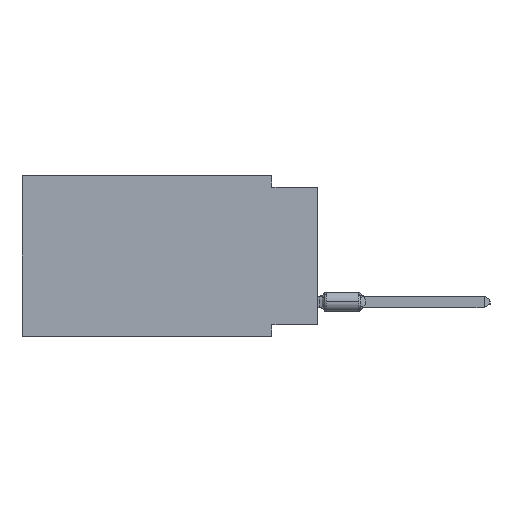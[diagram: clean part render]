
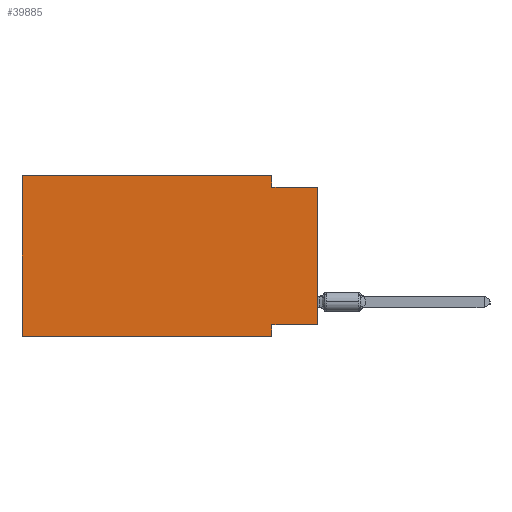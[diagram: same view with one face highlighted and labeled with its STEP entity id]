
A CAD part, left-side view. The second image highlights one B-rep face of the part: STEP entity #39885.
In plain terms, the highlighted planar face has unit normal (-1, 0, 0).
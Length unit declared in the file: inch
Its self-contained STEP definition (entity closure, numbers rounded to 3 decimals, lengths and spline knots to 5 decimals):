
#1700 = LINE ( 'NONE', #15161, #22522 ) ;
#3339 = CARTESIAN_POINT ( 'NONE',  ( 0., 0., -0.025 ) ) ;
#3641 = EDGE_CURVE ( 'NONE', #24175, #11158, #1700, .T. ) ;
#3850 = VERTEX_POINT ( 'NONE', #20729 ) ;
#4468 = EDGE_CURVE ( 'NONE', #24175, #17269, #24780, .T. ) ;
#5743 = EDGE_CURVE ( 'NONE', #25001, #36139, #16099, .T. ) ;
#5781 = DIRECTION ( 'NONE',  ( 1., 0., 0. ) ) ;
#6642 = VECTOR ( 'NONE', #9302, 39.37008 ) ;
#7160 = EDGE_CURVE ( 'NONE', #17269, #23336, #40997, .T. ) ;
#8405 = DIRECTION ( 'NONE',  ( 0., 0., -1. ) ) ;
#8498 = DIRECTION ( 'NONE',  ( 0., -1., 0. ) ) ;
#8763 = ORIENTED_EDGE ( 'NONE', *, *, #3641, .T. ) ;
#9302 = DIRECTION ( 'NONE',  ( 0., 0., -1. ) ) ;
#9422 = EDGE_CURVE ( 'NONE', #36139, #11158, #42247, .T. ) ;
#10622 = ORIENTED_EDGE ( 'NONE', *, *, #7160, .F. ) ;
#10647 = VECTOR ( 'NONE', #14175, 39.37008 ) ;
#10816 = CARTESIAN_POINT ( 'NONE',  ( 0., 0.645, 0. ) ) ;
#10922 = CARTESIAN_POINT ( 'NONE',  ( 0., 0., -0.325 ) ) ;
#10933 = CARTESIAN_POINT ( 'NONE',  ( 0., 0., 0. ) ) ;
#11158 = VERTEX_POINT ( 'NONE', #25811 ) ;
#12844 = LINE ( 'NONE', #18719, #37618 ) ;
#13560 = VECTOR ( 'NONE', #14609, 39.37008 ) ;
#13979 = EDGE_CURVE ( 'NONE', #3850, #23874, #12844, .T. ) ;
#14175 = DIRECTION ( 'NONE',  ( 0., 0., 1. ) ) ;
#14609 = DIRECTION ( 'NONE',  ( 0., 0., 1. ) ) ;
#15161 = CARTESIAN_POINT ( 'NONE',  ( 0., 0.645, -0.35 ) ) ;
#16099 = LINE ( 'NONE', #22815, #17570 ) ;
#17269 = VERTEX_POINT ( 'NONE', #10816 ) ;
#17570 = VECTOR ( 'NONE', #32368, 39.37008 ) ;
#17701 = LINE ( 'NONE', #20519, #39893 ) ;
#17793 = ORIENTED_EDGE ( 'NONE', *, *, #4468, .F. ) ;
#18469 = ORIENTED_EDGE ( 'NONE', *, *, #28599, .F. ) ;
#18719 = CARTESIAN_POINT ( 'NONE',  ( 0., 0., -0.025 ) ) ;
#20519 = CARTESIAN_POINT ( 'NONE',  ( 0., 0.1, 0. ) ) ;
#20729 = CARTESIAN_POINT ( 'NONE',  ( 0., 0.1, -0.025 ) ) ;
#21070 = ORIENTED_EDGE ( 'NONE', *, *, #23892, .T. ) ;
#21312 = CARTESIAN_POINT ( 'NONE',  ( 0., 0.645, 0. ) ) ;
#22246 = FACE_OUTER_BOUND ( 'NONE', #30746, .T. ) ;
#22522 = VECTOR ( 'NONE', #35082, 39.37008 ) ;
#22815 = CARTESIAN_POINT ( 'NONE',  ( 0., 0., -0.325 ) ) ;
#23336 = VERTEX_POINT ( 'NONE', #40030 ) ;
#23874 = VERTEX_POINT ( 'NONE', #3339 ) ;
#23892 = EDGE_CURVE ( 'NONE', #25001, #23874, #41029, .T. ) ;
#24175 = VERTEX_POINT ( 'NONE', #39918 ) ;
#24738 = CARTESIAN_POINT ( 'NONE',  ( 0., 0.645, 0. ) ) ;
#24780 = LINE ( 'NONE', #21312, #13560 ) ;
#25001 = VERTEX_POINT ( 'NONE', #10922 ) ;
#25061 = PLANE ( 'NONE',  #40151 ) ;
#25811 = CARTESIAN_POINT ( 'NONE',  ( 0., 0.1, -0.35 ) ) ;
#26498 = ORIENTED_EDGE ( 'NONE', *, *, #9422, .F. ) ;
#26510 = VECTOR ( 'NONE', #8498, 39.37008 ) ;
#26825 = DIRECTION ( 'NONE',  ( 0., 0., -1. ) ) ;
#28599 = EDGE_CURVE ( 'NONE', #23336, #3850, #17701, .T. ) ;
#30442 = ORIENTED_EDGE ( 'NONE', *, *, #13979, .F. ) ;
#30746 = EDGE_LOOP ( 'NONE', ( #21070, #30442, #18469, #10622, #17793, #8763, #26498, #34788 ) ) ;
#31922 = DIRECTION ( 'NONE',  ( 0., -1., 0. ) ) ;
#32368 = DIRECTION ( 'NONE',  ( 0., 1., 0. ) ) ;
#34788 = ORIENTED_EDGE ( 'NONE', *, *, #5743, .F. ) ;
#35082 = DIRECTION ( 'NONE',  ( 0., -1., 0. ) ) ;
#36139 = VERTEX_POINT ( 'NONE', #37499 ) ;
#37499 = CARTESIAN_POINT ( 'NONE',  ( 0., 0.1, -0.325 ) ) ;
#37618 = VECTOR ( 'NONE', #31922, 39.37008 ) ;
#39885 = ADVANCED_FACE ( 'NONE', ( #22246 ), #25061, .F. ) ;
#39893 = VECTOR ( 'NONE', #26825, 39.37008 ) ;
#39918 = CARTESIAN_POINT ( 'NONE',  ( 0., 0.645, -0.35 ) ) ;
#40030 = CARTESIAN_POINT ( 'NONE',  ( 0., 0.1, 0. ) ) ;
#40151 = AXIS2_PLACEMENT_3D ( 'NONE', #41774, #5781, #8405 ) ;
#40997 = LINE ( 'NONE', #24738, #26510 ) ;
#41029 = LINE ( 'NONE', #10933, #10647 ) ;
#41774 = CARTESIAN_POINT ( 'NONE',  ( 0., 0.645, 0. ) ) ;
#42247 = LINE ( 'NONE', #42876, #6642 ) ;
#42876 = CARTESIAN_POINT ( 'NONE',  ( 0., 0.1, -0.35 ) ) ;
